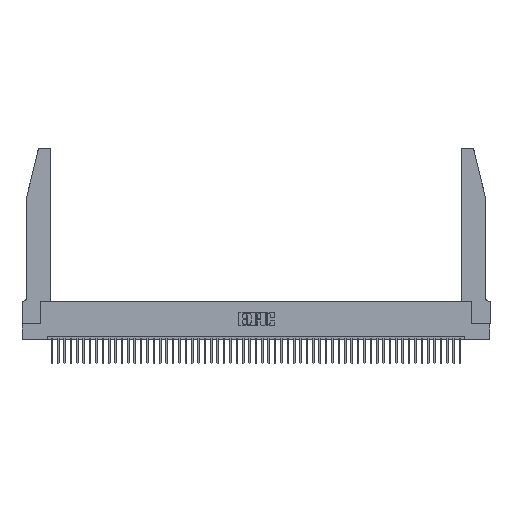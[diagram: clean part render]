
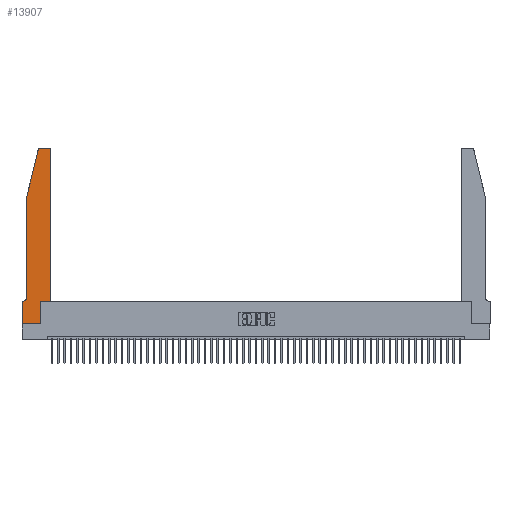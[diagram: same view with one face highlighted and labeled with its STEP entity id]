
A CAD part, top view. The second image highlights one B-rep face of the part: STEP entity #13907.
In plain terms, the highlighted planar face has unit normal (0, 0, 1).
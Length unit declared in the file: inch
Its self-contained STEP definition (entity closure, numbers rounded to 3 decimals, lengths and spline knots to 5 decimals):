
#174 = DIRECTION ( 'NONE',  ( -1., 0., 0. ) ) ;
#1740 = LINE ( 'NONE', #43861, #4931 ) ;
#1955 = DIRECTION ( 'NONE',  ( 0., -1., 0. ) ) ;
#2219 = LINE ( 'NONE', #19883, #4120 ) ;
#3668 = EDGE_CURVE ( 'NONE', #41084, #12679, #2219, .T. ) ;
#4120 = VECTOR ( 'NONE', #37263, 39.37008 ) ;
#4462 = EDGE_CURVE ( 'NONE', #35030, #4853, #20637, .T. ) ;
#4759 = DIRECTION ( 'NONE',  ( 1., 0., 0. ) ) ;
#4853 = VERTEX_POINT ( 'NONE', #25970 ) ;
#4931 = VECTOR ( 'NONE', #39072, 39.37008 ) ;
#7353 = ORIENTED_EDGE ( 'NONE', *, *, #3668, .T. ) ;
#7675 = DIRECTION ( 'NONE',  ( -0.239, -0.971, 0. ) ) ;
#7692 = EDGE_CURVE ( 'NONE', #26413, #32409, #12592, .T. ) ;
#8487 = VERTEX_POINT ( 'NONE', #30250 ) ;
#8798 = ORIENTED_EDGE ( 'NONE', *, *, #4462, .T. ) ;
#11380 = ORIENTED_EDGE ( 'NONE', *, *, #7692, .T. ) ;
#11953 = VERTEX_POINT ( 'NONE', #14933 ) ;
#12243 = LINE ( 'NONE', #52278, #49130 ) ;
#12592 = CIRCLE ( 'NONE', #18458, 0.03 ) ;
#12679 = VERTEX_POINT ( 'NONE', #15935 ) ;
#13045 = CARTESIAN_POINT ( 'NONE',  ( 0.284, 2.72, 0.37 ) ) ;
#13282 = ORIENTED_EDGE ( 'NONE', *, *, #16211, .T. ) ;
#13864 = AXIS2_PLACEMENT_3D ( 'NONE', #46284, #25692, #34552 ) ;
#13907 = ADVANCED_FACE ( 'NONE', ( #34891 ), #46643, .T. ) ;
#14433 = CARTESIAN_POINT ( 'NONE',  ( 0.0755, 2., 0.37 ) ) ;
#14933 = CARTESIAN_POINT ( 'NONE',  ( 0.0755, 0.42, 0.37 ) ) ;
#15935 = CARTESIAN_POINT ( 'NONE',  ( 0.2865, 0., 0.37 ) ) ;
#16095 = EDGE_CURVE ( 'NONE', #4853, #21924, #1740, .T. ) ;
#16211 = EDGE_CURVE ( 'NONE', #11953, #51999, #51361, .T. ) ;
#16410 = CARTESIAN_POINT ( 'NONE',  ( 0.2605, 2.75, 0.37 ) ) ;
#17153 = CARTESIAN_POINT ( 'NONE',  ( 0.284, 2.75, 0.37 ) ) ;
#17438 = LINE ( 'NONE', #16410, #21292 ) ;
#17744 = LINE ( 'NONE', #51289, #18361 ) ;
#18361 = VECTOR ( 'NONE', #39192, 39.37008 ) ;
#18458 = AXIS2_PLACEMENT_3D ( 'NONE', #13045, #42384, #28946 ) ;
#18787 = CARTESIAN_POINT ( 'NONE',  ( 0.0055, 0.35, 0.37 ) ) ;
#19883 = CARTESIAN_POINT ( 'NONE',  ( 0., 0., 0.37 ) ) ;
#20424 = VECTOR ( 'NONE', #1955, 39.37008 ) ;
#20637 = LINE ( 'NONE', #47155, #28280 ) ;
#21292 = VECTOR ( 'NONE', #174, 39.37008 ) ;
#21313 = VECTOR ( 'NONE', #7675, 39.37008 ) ;
#21424 = LINE ( 'NONE', #39557, #46838 ) ;
#21924 = VERTEX_POINT ( 'NONE', #42947 ) ;
#22778 = EDGE_CURVE ( 'NONE', #32409, #46210, #40353, .T. ) ;
#23575 = LINE ( 'NONE', #38428, #20424 ) ;
#24588 = VERTEX_POINT ( 'NONE', #40015 ) ;
#24845 = ORIENTED_EDGE ( 'NONE', *, *, #16095, .T. ) ;
#25692 = DIRECTION ( 'NONE',  ( 0., 0., 1. ) ) ;
#25970 = CARTESIAN_POINT ( 'NONE',  ( 0.4505, 0.35, 0.37 ) ) ;
#26047 = ORIENTED_EDGE ( 'NONE', *, *, #42194, .T. ) ;
#26413 = VERTEX_POINT ( 'NONE', #17153 ) ;
#27619 = EDGE_CURVE ( 'NONE', #21924, #24588, #51296, .T. ) ;
#28280 = VECTOR ( 'NONE', #46813, 39.37008 ) ;
#28946 = DIRECTION ( 'NONE',  ( 1., 0., 0. ) ) ;
#29057 = EDGE_LOOP ( 'NONE', ( #48407, #11380, #43250, #49228, #13282, #34949, #33831, #7353, #26047, #8798, #24845, #48487 ) ) ;
#29142 = DIRECTION ( 'NONE',  ( 0., 0., 1. ) ) ;
#29738 = EDGE_CURVE ( 'NONE', #24588, #26413, #17438, .T. ) ;
#30250 = CARTESIAN_POINT ( 'NONE',  ( 0., 0.35, 0.37 ) ) ;
#31673 = EDGE_CURVE ( 'NONE', #8487, #41084, #23575, .T. ) ;
#32409 = VERTEX_POINT ( 'NONE', #40850 ) ;
#32747 = EDGE_CURVE ( 'NONE', #46210, #11953, #17744, .T. ) ;
#33831 = ORIENTED_EDGE ( 'NONE', *, *, #31673, .T. ) ;
#34552 = DIRECTION ( 'NONE',  ( 1., 0., 0. ) ) ;
#34771 = CARTESIAN_POINT ( 'NONE',  ( 0.0755, 2., 0.37 ) ) ;
#34891 = FACE_OUTER_BOUND ( 'NONE', #29057, .T. ) ;
#34949 = ORIENTED_EDGE ( 'NONE', *, *, #46234, .T. ) ;
#35030 = VERTEX_POINT ( 'NONE', #41558 ) ;
#35287 = DIRECTION ( 'NONE',  ( -1., 0., 0. ) ) ;
#37263 = DIRECTION ( 'NONE',  ( 1., 0., 0. ) ) ;
#38428 = CARTESIAN_POINT ( 'NONE',  ( 0., 0., 0.37 ) ) ;
#39072 = DIRECTION ( 'NONE',  ( 0., 1., 0. ) ) ;
#39192 = DIRECTION ( 'NONE',  ( 0., -1., 0. ) ) ;
#39557 = CARTESIAN_POINT ( 'NONE',  ( 0.0755, 0.35, 0.37 ) ) ;
#40015 = CARTESIAN_POINT ( 'NONE',  ( 0.4205, 2.75, 0.37 ) ) ;
#40353 = LINE ( 'NONE', #14433, #21313 ) ;
#40850 = CARTESIAN_POINT ( 'NONE',  ( 0.25487, 2.72718, 0.37 ) ) ;
#41084 = VERTEX_POINT ( 'NONE', #45305 ) ;
#41558 = CARTESIAN_POINT ( 'NONE',  ( 0.2865, 0.35, 0.37 ) ) ;
#42194 = EDGE_CURVE ( 'NONE', #12679, #35030, #12243, .T. ) ;
#42384 = DIRECTION ( 'NONE',  ( 0., 0., 1. ) ) ;
#42947 = CARTESIAN_POINT ( 'NONE',  ( 0.4505, 2.72, 0.37 ) ) ;
#43250 = ORIENTED_EDGE ( 'NONE', *, *, #22778, .T. ) ;
#43861 = CARTESIAN_POINT ( 'NONE',  ( 0.4505, 0.35, 0.37 ) ) ;
#43951 = DIRECTION ( 'NONE',  ( 0., 1., 0. ) ) ;
#44039 = DIRECTION ( 'NONE',  ( -1., 0., 0. ) ) ;
#44217 = CARTESIAN_POINT ( 'NONE',  ( 0.0055, 0.42, 0.37 ) ) ;
#45305 = CARTESIAN_POINT ( 'NONE',  ( 0., 0., 0.37 ) ) ;
#45656 = CARTESIAN_POINT ( 'NONE',  ( 0.4205, 2.72, 0.37 ) ) ;
#46210 = VERTEX_POINT ( 'NONE', #34771 ) ;
#46234 = EDGE_CURVE ( 'NONE', #51999, #8487, #21424, .T. ) ;
#46284 = CARTESIAN_POINT ( 'NONE',  ( 0., 0.35, 0.37 ) ) ;
#46643 = PLANE ( 'NONE',  #13864 ) ;
#46813 = DIRECTION ( 'NONE',  ( 1., 0., 0. ) ) ;
#46838 = VECTOR ( 'NONE', #35287, 39.37008 ) ;
#47155 = CARTESIAN_POINT ( 'NONE',  ( 0.4505, 0.35, 0.37 ) ) ;
#47323 = AXIS2_PLACEMENT_3D ( 'NONE', #44217, #48082, #44039 ) ;
#48082 = DIRECTION ( 'NONE',  ( 0., 0., -1. ) ) ;
#48407 = ORIENTED_EDGE ( 'NONE', *, *, #29738, .T. ) ;
#48487 = ORIENTED_EDGE ( 'NONE', *, *, #27619, .T. ) ;
#49130 = VECTOR ( 'NONE', #43951, 39.37008 ) ;
#49228 = ORIENTED_EDGE ( 'NONE', *, *, #32747, .T. ) ;
#51289 = CARTESIAN_POINT ( 'NONE',  ( 0.0755, 2., 0.37 ) ) ;
#51296 = CIRCLE ( 'NONE', #52079, 0.03 ) ;
#51361 = CIRCLE ( 'NONE', #47323, 0.07 ) ;
#51999 = VERTEX_POINT ( 'NONE', #18787 ) ;
#52079 = AXIS2_PLACEMENT_3D ( 'NONE', #45656, #29142, #4759 ) ;
#52278 = CARTESIAN_POINT ( 'NONE',  ( 0.2865, 0.35, 0.37 ) ) ;
